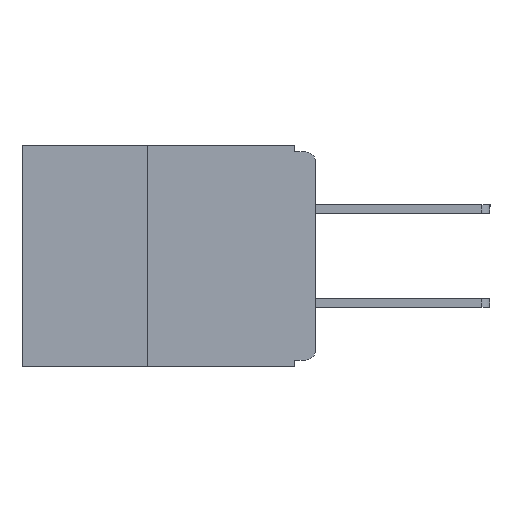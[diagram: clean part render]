
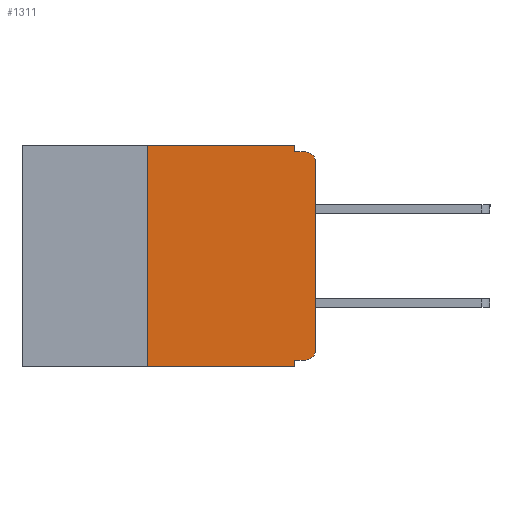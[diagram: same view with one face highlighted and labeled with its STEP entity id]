
A CAD part, left-side view. The second image highlights one B-rep face of the part: STEP entity #1311.
In plain terms, the highlighted planar face has unit normal (-1, 0, 0).
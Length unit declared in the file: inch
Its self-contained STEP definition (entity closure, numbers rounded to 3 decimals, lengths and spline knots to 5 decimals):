
#11 = ORIENTED_EDGE ( 'NONE', *, *, #7965, .F. ) ;
#310 = CIRCLE ( 'NONE', #5345, 0.015 ) ;
#377 = VERTEX_POINT ( 'NONE', #6210 ) ;
#510 = EDGE_CURVE ( 'NONE', #13365, #377, #2356, .T. ) ;
#769 = VECTOR ( 'NONE', #14449, 39.37008 ) ;
#844 = CARTESIAN_POINT ( 'NONE',  ( 0., 0., -0.32 ) ) ;
#926 = EDGE_CURVE ( 'NONE', #7930, #6961, #12387, .T. ) ;
#932 = LINE ( 'NONE', #2678, #4257 ) ;
#942 = FACE_OUTER_BOUND ( 'NONE', #12255, .T. ) ;
#1067 = VECTOR ( 'NONE', #5193, 39.37008 ) ;
#1151 = CARTESIAN_POINT ( 'NONE',  ( 0., 0.031, -0.33 ) ) ;
#1311 = ADVANCED_FACE ( 'NONE', ( #942 ), #3100, .F. ) ;
#1555 = AXIS2_PLACEMENT_3D ( 'NONE', #8537, #8562, #12293 ) ;
#1868 = CARTESIAN_POINT ( 'NONE',  ( 0., 0., 0. ) ) ;
#1987 = VERTEX_POINT ( 'NONE', #6939 ) ;
#2072 = CARTESIAN_POINT ( 'NONE',  ( 0., 0.015, -0.305 ) ) ;
#2356 = LINE ( 'NONE', #4578, #8425 ) ;
#2579 = ORIENTED_EDGE ( 'NONE', *, *, #15520, .T. ) ;
#2678 = CARTESIAN_POINT ( 'NONE',  ( 0., 0.25, -0.33 ) ) ;
#2738 = VECTOR ( 'NONE', #8151, 39.37008 ) ;
#3100 = PLANE ( 'NONE',  #1555 ) ;
#3155 = ORIENTED_EDGE ( 'NONE', *, *, #510, .F. ) ;
#3315 = DIRECTION ( 'NONE',  ( 0., 0., -1. ) ) ;
#3534 = VECTOR ( 'NONE', #8167, 39.37008 ) ;
#3784 = CARTESIAN_POINT ( 'NONE',  ( 0., 0., -0.305 ) ) ;
#4257 = VECTOR ( 'NONE', #12352, 39.37008 ) ;
#4466 = LINE ( 'NONE', #1151, #769 ) ;
#4578 = CARTESIAN_POINT ( 'NONE',  ( 0., 0., -0.01 ) ) ;
#4763 = LINE ( 'NONE', #11202, #1067 ) ;
#5025 = EDGE_CURVE ( 'NONE', #6156, #377, #11555, .T. ) ;
#5162 = LINE ( 'NONE', #1868, #7973 ) ;
#5193 = DIRECTION ( 'NONE',  ( 0., -1., 0. ) ) ;
#5345 = AXIS2_PLACEMENT_3D ( 'NONE', #2072, #10587, #3315 ) ;
#5672 = CARTESIAN_POINT ( 'NONE',  ( 0., 0.031, -0.01 ) ) ;
#6062 = ORIENTED_EDGE ( 'NONE', *, *, #14724, .F. ) ;
#6156 = VERTEX_POINT ( 'NONE', #12413 ) ;
#6210 = CARTESIAN_POINT ( 'NONE',  ( 0., 0.015, -0.01 ) ) ;
#6220 = ORIENTED_EDGE ( 'NONE', *, *, #5025, .T. ) ;
#6316 = CARTESIAN_POINT ( 'NONE',  ( 0., 0.437, 0. ) ) ;
#6544 = ORIENTED_EDGE ( 'NONE', *, *, #15125, .T. ) ;
#6748 = CARTESIAN_POINT ( 'NONE',  ( 0., 0.031, -0.32 ) ) ;
#6939 = CARTESIAN_POINT ( 'NONE',  ( 0., 0.25, -0.33 ) ) ;
#6961 = VERTEX_POINT ( 'NONE', #10964 ) ;
#6986 = VERTEX_POINT ( 'NONE', #3784 ) ;
#7311 = CARTESIAN_POINT ( 'NONE',  ( 0., 0.031, 0. ) ) ;
#7339 = VERTEX_POINT ( 'NONE', #14122 ) ;
#7344 = ORIENTED_EDGE ( 'NONE', *, *, #15058, .T. ) ;
#7686 = ORIENTED_EDGE ( 'NONE', *, *, #12926, .F. ) ;
#7930 = VERTEX_POINT ( 'NONE', #10522 ) ;
#7965 = EDGE_CURVE ( 'NONE', #7339, #14426, #10007, .T. ) ;
#7973 = VECTOR ( 'NONE', #15131, 39.37008 ) ;
#8151 = DIRECTION ( 'NONE',  ( 0., -1., 0. ) ) ;
#8167 = DIRECTION ( 'NONE',  ( 0., 1., 0. ) ) ;
#8425 = VECTOR ( 'NONE', #13498, 39.37008 ) ;
#8452 = ORIENTED_EDGE ( 'NONE', *, *, #13574, .F. ) ;
#8512 = AXIS2_PLACEMENT_3D ( 'NONE', #12448, #12431, #12397 ) ;
#8537 = CARTESIAN_POINT ( 'NONE',  ( 0., 0.437, 0. ) ) ;
#8562 = DIRECTION ( 'NONE',  ( 1., 0., 0. ) ) ;
#10007 = LINE ( 'NONE', #844, #3534 ) ;
#10105 = LINE ( 'NONE', #7311, #13611 ) ;
#10522 = CARTESIAN_POINT ( 'NONE',  ( 0., 0.25, 0. ) ) ;
#10587 = DIRECTION ( 'NONE',  ( -1., 0., 0. ) ) ;
#10713 = CARTESIAN_POINT ( 'NONE',  ( 0., 0.031, -0.33 ) ) ;
#10964 = CARTESIAN_POINT ( 'NONE',  ( 0., 0.031, 0. ) ) ;
#11202 = CARTESIAN_POINT ( 'NONE',  ( 0., 0.437, -0.33 ) ) ;
#11555 = CIRCLE ( 'NONE', #8512, 0.015 ) ;
#11735 = VERTEX_POINT ( 'NONE', #10713 ) ;
#12255 = EDGE_LOOP ( 'NONE', ( #7344, #6220, #3155, #6062, #13576, #8452, #2579, #7686, #11, #6544 ) ) ;
#12293 = DIRECTION ( 'NONE',  ( 0., 0., -1. ) ) ;
#12352 = DIRECTION ( 'NONE',  ( 0., 0., 1. ) ) ;
#12387 = LINE ( 'NONE', #6316, #2738 ) ;
#12397 = DIRECTION ( 'NONE',  ( 0., 0., -1. ) ) ;
#12413 = CARTESIAN_POINT ( 'NONE',  ( 0., 0., -0.025 ) ) ;
#12431 = DIRECTION ( 'NONE',  ( -1., 0., 0. ) ) ;
#12448 = CARTESIAN_POINT ( 'NONE',  ( 0., 0.015, -0.025 ) ) ;
#12926 = EDGE_CURVE ( 'NONE', #14426, #11735, #4466, .T. ) ;
#13365 = VERTEX_POINT ( 'NONE', #5672 ) ;
#13498 = DIRECTION ( 'NONE',  ( 0., -1., 0. ) ) ;
#13574 = EDGE_CURVE ( 'NONE', #1987, #7930, #932, .T. ) ;
#13576 = ORIENTED_EDGE ( 'NONE', *, *, #926, .F. ) ;
#13611 = VECTOR ( 'NONE', #15701, 39.37008 ) ;
#14122 = CARTESIAN_POINT ( 'NONE',  ( 0., 0.015, -0.32 ) ) ;
#14426 = VERTEX_POINT ( 'NONE', #6748 ) ;
#14449 = DIRECTION ( 'NONE',  ( 0., 0., -1. ) ) ;
#14724 = EDGE_CURVE ( 'NONE', #6961, #13365, #10105, .T. ) ;
#15058 = EDGE_CURVE ( 'NONE', #6986, #6156, #5162, .T. ) ;
#15125 = EDGE_CURVE ( 'NONE', #7339, #6986, #310, .T. ) ;
#15131 = DIRECTION ( 'NONE',  ( 0., 0., 1. ) ) ;
#15520 = EDGE_CURVE ( 'NONE', #1987, #11735, #4763, .T. ) ;
#15701 = DIRECTION ( 'NONE',  ( 0., 0., -1. ) ) ;
